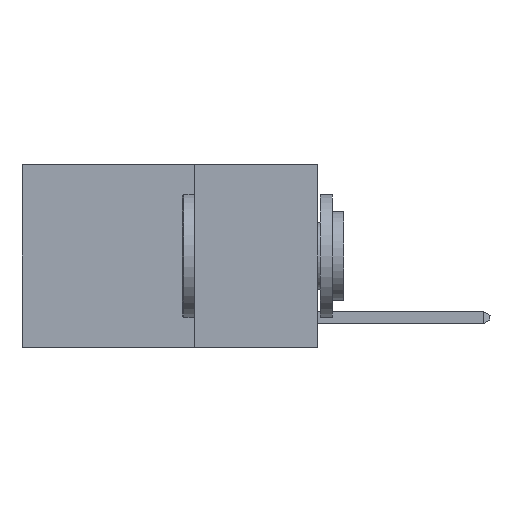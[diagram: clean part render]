
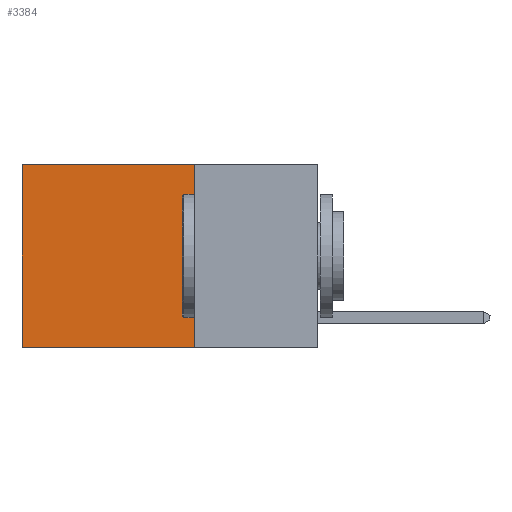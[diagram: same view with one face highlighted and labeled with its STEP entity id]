
A CAD part, left-side view. The second image highlights one B-rep face of the part: STEP entity #3384.
In plain terms, the highlighted planar face has unit normal (-1, 0, 0).
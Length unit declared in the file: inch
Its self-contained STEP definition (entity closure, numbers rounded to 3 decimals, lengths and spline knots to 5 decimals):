
#50 = CARTESIAN_POINT ( 'NONE',  ( 0.2625, 0.25, 0. ) ) ;
#126 = EDGE_CURVE ( 'NONE', #2287, #289, #623, .T. ) ;
#167 = LINE ( 'NONE', #4082, #6121 ) ;
#289 = VERTEX_POINT ( 'NONE', #4250 ) ;
#606 = VECTOR ( 'NONE', #11249, 39.37008 ) ;
#612 = EDGE_CURVE ( 'NONE', #2287, #12783, #2858, .T. ) ;
#623 = LINE ( 'NONE', #4596, #11259 ) ;
#1055 = PLANE ( 'NONE',  #1289 ) ;
#1289 = AXIS2_PLACEMENT_3D ( 'NONE', #50, #7214, #12140 ) ;
#2287 = VERTEX_POINT ( 'NONE', #11885 ) ;
#2858 = LINE ( 'NONE', #5906, #7134 ) ;
#3186 = FACE_OUTER_BOUND ( 'NONE', #4106, .T. ) ;
#3384 = ADVANCED_FACE ( 'NONE', ( #3186 ), #1055, .F. ) ;
#4082 = CARTESIAN_POINT ( 'NONE',  ( 0.2625, 0.6, 0. ) ) ;
#4106 = EDGE_LOOP ( 'NONE', ( #12184, #4122, #10948, #5845 ) ) ;
#4122 = ORIENTED_EDGE ( 'NONE', *, *, #5746, .F. ) ;
#4250 = CARTESIAN_POINT ( 'NONE',  ( 0.2625, 0.6, 0. ) ) ;
#4382 = CARTESIAN_POINT ( 'NONE',  ( 0.2625, 0.6, -0.37 ) ) ;
#4596 = CARTESIAN_POINT ( 'NONE',  ( 0.2625, 0.25, 0. ) ) ;
#5182 = LINE ( 'NONE', #11119, #606 ) ;
#5746 = EDGE_CURVE ( 'NONE', #12783, #7591, #5182, .T. ) ;
#5845 = ORIENTED_EDGE ( 'NONE', *, *, #126, .T. ) ;
#5906 = CARTESIAN_POINT ( 'NONE',  ( 0.2625, 0.25, 0. ) ) ;
#6121 = VECTOR ( 'NONE', #12257, 39.37008 ) ;
#6663 = DIRECTION ( 'NONE',  ( 0., 1., 0. ) ) ;
#6967 = CARTESIAN_POINT ( 'NONE',  ( 0.2625, 0.25, -0.37 ) ) ;
#7134 = VECTOR ( 'NONE', #10967, 39.37008 ) ;
#7214 = DIRECTION ( 'NONE',  ( 1., 0., 0. ) ) ;
#7591 = VERTEX_POINT ( 'NONE', #4382 ) ;
#8489 = EDGE_CURVE ( 'NONE', #289, #7591, #167, .T. ) ;
#10948 = ORIENTED_EDGE ( 'NONE', *, *, #612, .F. ) ;
#10967 = DIRECTION ( 'NONE',  ( 0., 0., -1. ) ) ;
#11119 = CARTESIAN_POINT ( 'NONE',  ( 0.2625, 0.25, -0.37 ) ) ;
#11249 = DIRECTION ( 'NONE',  ( 0., 1., 0. ) ) ;
#11259 = VECTOR ( 'NONE', #6663, 39.37008 ) ;
#11885 = CARTESIAN_POINT ( 'NONE',  ( 0.2625, 0.25, 0. ) ) ;
#12140 = DIRECTION ( 'NONE',  ( 0., 0., -1. ) ) ;
#12184 = ORIENTED_EDGE ( 'NONE', *, *, #8489, .T. ) ;
#12257 = DIRECTION ( 'NONE',  ( 0., 0., -1. ) ) ;
#12783 = VERTEX_POINT ( 'NONE', #6967 ) ;
